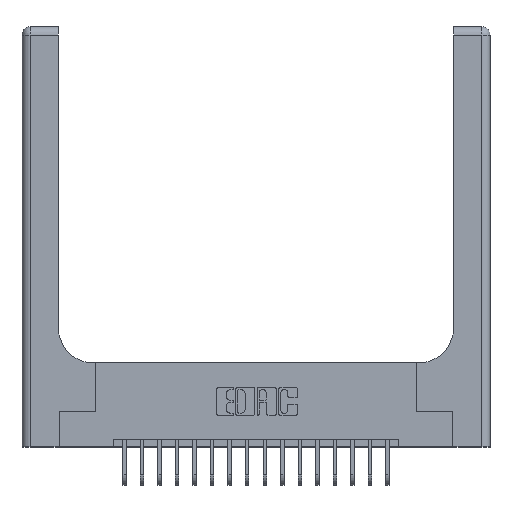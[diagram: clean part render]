
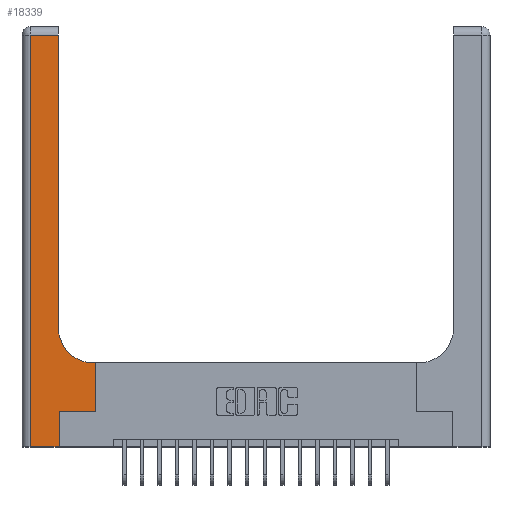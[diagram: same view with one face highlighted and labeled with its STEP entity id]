
A CAD part, top view. The second image highlights one B-rep face of the part: STEP entity #18339.
In plain terms, the highlighted planar face has unit normal (0, 0, 1).
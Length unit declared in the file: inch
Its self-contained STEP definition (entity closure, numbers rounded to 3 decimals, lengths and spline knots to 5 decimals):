
#470 = EDGE_CURVE ( 'NONE', #9269, #6471, #2293, .T. ) ;
#560 = DIRECTION ( 'NONE',  ( 1., 0., 0. ) ) ;
#682 = VECTOR ( 'NONE', #560, 39.37008 ) ;
#1086 = VERTEX_POINT ( 'NONE', #4994 ) ;
#2293 = LINE ( 'NONE', #16989, #682 ) ;
#2494 = CARTESIAN_POINT ( 'NONE',  ( 0.528, 0.25, 0.37 ) ) ;
#2518 = CARTESIAN_POINT ( 'NONE',  ( 0.528, 0.6, 0.37 ) ) ;
#2760 = DIRECTION ( 'NONE',  ( -1., 0., 0. ) ) ;
#3092 = CARTESIAN_POINT ( 'NONE',  ( 0.26, 0.6, 0.37 ) ) ;
#3681 = EDGE_LOOP ( 'NONE', ( #8566, #20861, #19639, #8930, #7200, #6946, #17469, #17612, #15930 ) ) ;
#4286 = DIRECTION ( 'NONE',  ( 0., -1., 0. ) ) ;
#4348 = VECTOR ( 'NONE', #8606, 39.37008 ) ;
#4717 = CARTESIAN_POINT ( 'NONE',  ( 0.26, 0.85, 0.37 ) ) ;
#4975 = CARTESIAN_POINT ( 'NONE',  ( 0.265, 0., 0.37 ) ) ;
#4994 = CARTESIAN_POINT ( 'NONE',  ( 0.26, 2.94, 0.37 ) ) ;
#5267 = CARTESIAN_POINT ( 'NONE',  ( 0.26, 3., 0.37 ) ) ;
#5354 = AXIS2_PLACEMENT_3D ( 'NONE', #12888, #14388, #12458 ) ;
#5498 = EDGE_CURVE ( 'NONE', #11172, #1086, #20051, .T. ) ;
#5798 = DIRECTION ( 'NONE',  ( 1., 0., 0. ) ) ;
#6471 = VERTEX_POINT ( 'NONE', #20421 ) ;
#6670 = CARTESIAN_POINT ( 'NONE',  ( 0., 2.94, 0.37 ) ) ;
#6823 = EDGE_CURVE ( 'NONE', #10627, #9269, #18352, .T. ) ;
#6946 = ORIENTED_EDGE ( 'NONE', *, *, #14977, .T. ) ;
#6972 = EDGE_CURVE ( 'NONE', #16548, #12092, #7988, .T. ) ;
#7200 = ORIENTED_EDGE ( 'NONE', *, *, #20921, .T. ) ;
#7269 = LINE ( 'NONE', #13821, #16045 ) ;
#7914 = CARTESIAN_POINT ( 'NONE',  ( 0.06, 2.94, 0.37 ) ) ;
#7988 = LINE ( 'NONE', #3092, #15532 ) ;
#8566 = ORIENTED_EDGE ( 'NONE', *, *, #5498, .T. ) ;
#8606 = DIRECTION ( 'NONE',  ( -1., 0., 0. ) ) ;
#8758 = CARTESIAN_POINT ( 'NONE',  ( 0.06, 0., 0.37 ) ) ;
#8930 = ORIENTED_EDGE ( 'NONE', *, *, #470, .T. ) ;
#9251 = FACE_OUTER_BOUND ( 'NONE', #3681, .T. ) ;
#9269 = VERTEX_POINT ( 'NONE', #8758 ) ;
#9568 = CARTESIAN_POINT ( 'NONE',  ( 0.265, 0.25, 0.37 ) ) ;
#10172 = CARTESIAN_POINT ( 'NONE',  ( 0.06, 3., 0.37 ) ) ;
#10627 = VERTEX_POINT ( 'NONE', #7914 ) ;
#11172 = VERTEX_POINT ( 'NONE', #4717 ) ;
#11260 = DIRECTION ( 'NONE',  ( 0., 1., 0. ) ) ;
#11283 = CIRCLE ( 'NONE', #16436, 0.25 ) ;
#11534 = DIRECTION ( 'NONE',  ( 0., 1., 0. ) ) ;
#12092 = VERTEX_POINT ( 'NONE', #19878 ) ;
#12363 = CARTESIAN_POINT ( 'NONE',  ( 0.51, 0.85, 0.37 ) ) ;
#12458 = DIRECTION ( 'NONE',  ( -1., 0., 0. ) ) ;
#12516 = DIRECTION ( 'NONE',  ( 0., 1., 0. ) ) ;
#12884 = LINE ( 'NONE', #9568, #18048 ) ;
#12888 = CARTESIAN_POINT ( 'NONE',  ( 0., 3., 0.37 ) ) ;
#13821 = CARTESIAN_POINT ( 'NONE',  ( 0.528, 0.25, 0.37 ) ) ;
#14388 = DIRECTION ( 'NONE',  ( 0., 0., -1. ) ) ;
#14793 = VECTOR ( 'NONE', #11260, 39.37008 ) ;
#14977 = EDGE_CURVE ( 'NONE', #19320, #17070, #12884, .T. ) ;
#15532 = VECTOR ( 'NONE', #2760, 39.37008 ) ;
#15930 = ORIENTED_EDGE ( 'NONE', *, *, #19566, .T. ) ;
#16045 = VECTOR ( 'NONE', #12516, 39.37008 ) ;
#16436 = AXIS2_PLACEMENT_3D ( 'NONE', #12363, #17089, #5798 ) ;
#16548 = VERTEX_POINT ( 'NONE', #2518 ) ;
#16989 = CARTESIAN_POINT ( 'NONE',  ( 0., 0., 0.37 ) ) ;
#17070 = VERTEX_POINT ( 'NONE', #2494 ) ;
#17089 = DIRECTION ( 'NONE',  ( 0., 0., -1. ) ) ;
#17469 = ORIENTED_EDGE ( 'NONE', *, *, #21094, .T. ) ;
#17612 = ORIENTED_EDGE ( 'NONE', *, *, #6972, .T. ) ;
#17827 = DIRECTION ( 'NONE',  ( 1., 0., 0. ) ) ;
#17858 = CARTESIAN_POINT ( 'NONE',  ( 0.265, 0.25, 0.37 ) ) ;
#18048 = VECTOR ( 'NONE', #17827, 39.37008 ) ;
#18132 = VECTOR ( 'NONE', #11534, 39.37008 ) ;
#18339 = ADVANCED_FACE ( 'NONE', ( #9251 ), #19243, .F. ) ;
#18352 = LINE ( 'NONE', #10172, #19330 ) ;
#19243 = PLANE ( 'NONE',  #5354 ) ;
#19320 = VERTEX_POINT ( 'NONE', #17858 ) ;
#19330 = VECTOR ( 'NONE', #4286, 39.37008 ) ;
#19339 = EDGE_CURVE ( 'NONE', #1086, #10627, #19920, .T. ) ;
#19439 = LINE ( 'NONE', #4975, #14793 ) ;
#19566 = EDGE_CURVE ( 'NONE', #12092, #11172, #11283, .T. ) ;
#19639 = ORIENTED_EDGE ( 'NONE', *, *, #6823, .T. ) ;
#19878 = CARTESIAN_POINT ( 'NONE',  ( 0.51, 0.6, 0.37 ) ) ;
#19920 = LINE ( 'NONE', #6670, #4348 ) ;
#20051 = LINE ( 'NONE', #5267, #18132 ) ;
#20421 = CARTESIAN_POINT ( 'NONE',  ( 0.265, 0., 0.37 ) ) ;
#20861 = ORIENTED_EDGE ( 'NONE', *, *, #19339, .T. ) ;
#20921 = EDGE_CURVE ( 'NONE', #6471, #19320, #19439, .T. ) ;
#21094 = EDGE_CURVE ( 'NONE', #17070, #16548, #7269, .T. ) ;
